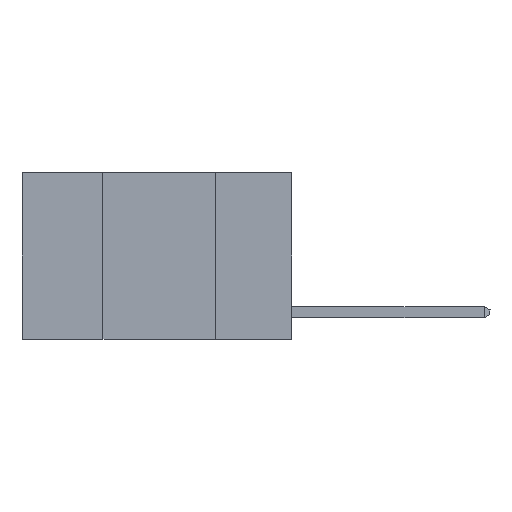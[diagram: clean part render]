
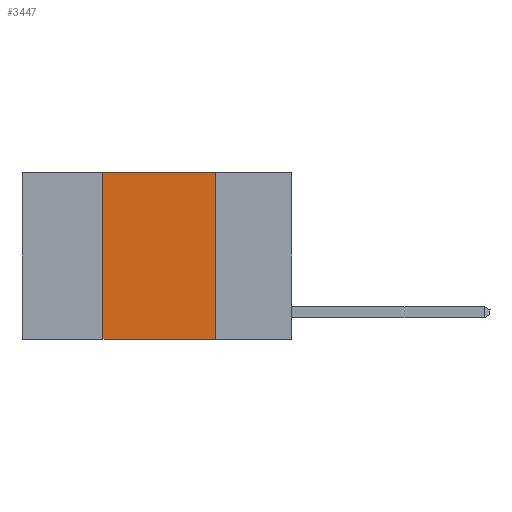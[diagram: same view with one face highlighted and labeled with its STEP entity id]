
A CAD part, left-side view. The second image highlights one B-rep face of the part: STEP entity #3447.
In plain terms, the highlighted planar face has unit normal (-1, 0, 0).
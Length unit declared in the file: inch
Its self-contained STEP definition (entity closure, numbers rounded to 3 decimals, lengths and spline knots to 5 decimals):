
#186 = VECTOR ( 'NONE', #1587, 39.37008 ) ;
#249 = FACE_OUTER_BOUND ( 'NONE', #6334, .T. ) ;
#425 = ORIENTED_EDGE ( 'NONE', *, *, #11929, .F. ) ;
#457 = ORIENTED_EDGE ( 'NONE', *, *, #12799, .F. ) ;
#540 = ORIENTED_EDGE ( 'NONE', *, *, #15212, .F. ) ;
#562 = ORIENTED_EDGE ( 'NONE', *, *, #5244, .T. ) ;
#1587 = DIRECTION ( 'NONE',  ( 0., 0., 1. ) ) ;
#1661 = VERTEX_POINT ( 'NONE', #14793 ) ;
#2023 = CARTESIAN_POINT ( 'NONE',  ( 0., 0.17, 0. ) ) ;
#2180 = AXIS2_PLACEMENT_3D ( 'NONE', #12744, #12485, #12423 ) ;
#3447 = ADVANCED_FACE ( 'NONE', ( #249 ), #12969, .F. ) ;
#3571 = LINE ( 'NONE', #7821, #186 ) ;
#3944 = CARTESIAN_POINT ( 'NONE',  ( 0., 0.6, 0. ) ) ;
#4489 = VECTOR ( 'NONE', #5775, 39.37008 ) ;
#4725 = VECTOR ( 'NONE', #15086, 39.37008 ) ;
#5244 = EDGE_CURVE ( 'NONE', #1661, #13585, #11150, .T. ) ;
#5775 = DIRECTION ( 'NONE',  ( 0., 0., -1. ) ) ;
#6334 = EDGE_LOOP ( 'NONE', ( #425, #457, #540, #562 ) ) ;
#7821 = CARTESIAN_POINT ( 'NONE',  ( 0., 0.42, 0. ) ) ;
#9736 = VECTOR ( 'NONE', #14636, 39.37008 ) ;
#10501 = CARTESIAN_POINT ( 'NONE',  ( 0., 0.6, -0.37 ) ) ;
#11150 = LINE ( 'NONE', #10501, #4725 ) ;
#11704 = CARTESIAN_POINT ( 'NONE',  ( 0., 0.17, 0. ) ) ;
#11929 = EDGE_CURVE ( 'NONE', #13381, #13585, #13986, .T. ) ;
#12369 = CARTESIAN_POINT ( 'NONE',  ( 0., 0.42, 0. ) ) ;
#12423 = DIRECTION ( 'NONE',  ( 0., 0., -1. ) ) ;
#12485 = DIRECTION ( 'NONE',  ( 1., 0., 0. ) ) ;
#12744 = CARTESIAN_POINT ( 'NONE',  ( 0., 0.6, 0. ) ) ;
#12799 = EDGE_CURVE ( 'NONE', #15072, #13381, #12833, .T. ) ;
#12833 = LINE ( 'NONE', #3944, #9736 ) ;
#12969 = PLANE ( 'NONE',  #2180 ) ;
#13381 = VERTEX_POINT ( 'NONE', #11704 ) ;
#13535 = CARTESIAN_POINT ( 'NONE',  ( 0., 0.17, -0.37 ) ) ;
#13585 = VERTEX_POINT ( 'NONE', #13535 ) ;
#13986 = LINE ( 'NONE', #2023, #4489 ) ;
#14636 = DIRECTION ( 'NONE',  ( 0., -1., 0. ) ) ;
#14793 = CARTESIAN_POINT ( 'NONE',  ( 0., 0.42, -0.37 ) ) ;
#15072 = VERTEX_POINT ( 'NONE', #12369 ) ;
#15086 = DIRECTION ( 'NONE',  ( 0., -1., 0. ) ) ;
#15212 = EDGE_CURVE ( 'NONE', #1661, #15072, #3571, .T. ) ;
